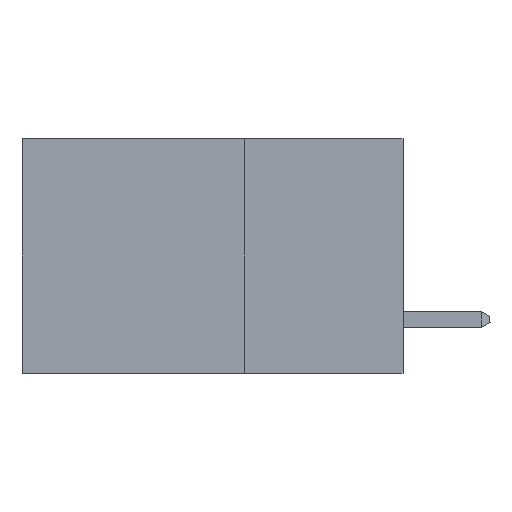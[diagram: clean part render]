
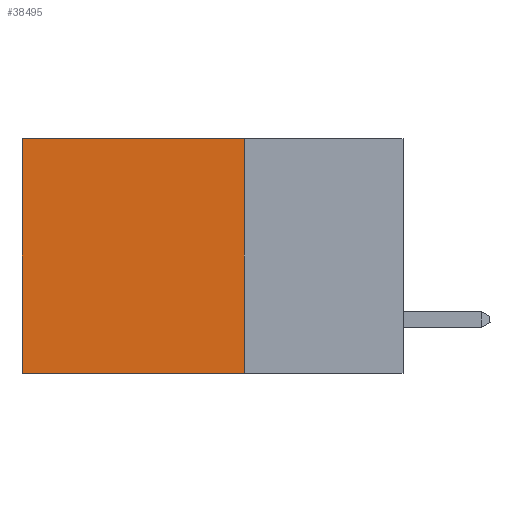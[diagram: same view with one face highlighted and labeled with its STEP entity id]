
A CAD part, left-side view. The second image highlights one B-rep face of the part: STEP entity #38495.
In plain terms, the highlighted planar face has unit normal (-1, 0, 0).
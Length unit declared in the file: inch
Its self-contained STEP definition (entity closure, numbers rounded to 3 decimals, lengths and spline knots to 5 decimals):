
#2037 = PLANE ( 'NONE',  #40340 ) ;
#2055 = CARTESIAN_POINT ( 'NONE',  ( 0.2875, 0.25, 0. ) ) ;
#2786 = VERTEX_POINT ( 'NONE', #8508 ) ;
#3442 = FACE_OUTER_BOUND ( 'NONE', #38806, .T. ) ;
#3471 = CARTESIAN_POINT ( 'NONE',  ( 0.2875, 0.25, 0. ) ) ;
#4425 = VECTOR ( 'NONE', #43375, 39.37008 ) ;
#5122 = EDGE_CURVE ( 'NONE', #25894, #33796, #31458, .T. ) ;
#5838 = CARTESIAN_POINT ( 'NONE',  ( 0.2875, 0.25, 0. ) ) ;
#7731 = CARTESIAN_POINT ( 'NONE',  ( 0.2875, 0.6, 0. ) ) ;
#8087 = ORIENTED_EDGE ( 'NONE', *, *, #5122, .F. ) ;
#8508 = CARTESIAN_POINT ( 'NONE',  ( 0.2875, 0.6, -0.37 ) ) ;
#11336 = VECTOR ( 'NONE', #37614, 39.37008 ) ;
#13285 = DIRECTION ( 'NONE',  ( 1., 0., 0. ) ) ;
#15306 = CARTESIAN_POINT ( 'NONE',  ( 0.2875, 0.25, -0.37 ) ) ;
#16373 = DIRECTION ( 'NONE',  ( 0., 1., 0. ) ) ;
#16949 = DIRECTION ( 'NONE',  ( 0., 0., -1. ) ) ;
#21003 = LINE ( 'NONE', #5838, #4425 ) ;
#25248 = ORIENTED_EDGE ( 'NONE', *, *, #46511, .T. ) ;
#25894 = VERTEX_POINT ( 'NONE', #2055 ) ;
#26436 = VECTOR ( 'NONE', #16373, 39.37008 ) ;
#28484 = CARTESIAN_POINT ( 'NONE',  ( 0.2875, 0.25, 0. ) ) ;
#30358 = VERTEX_POINT ( 'NONE', #7731 ) ;
#31458 = LINE ( 'NONE', #3471, #11336 ) ;
#33796 = VERTEX_POINT ( 'NONE', #15306 ) ;
#33809 = ORIENTED_EDGE ( 'NONE', *, *, #45675, .F. ) ;
#34390 = EDGE_CURVE ( 'NONE', #30358, #2786, #45422, .T. ) ;
#37614 = DIRECTION ( 'NONE',  ( 0., 0., -1. ) ) ;
#38005 = CARTESIAN_POINT ( 'NONE',  ( 0.2875, 0.6, 0. ) ) ;
#38495 = ADVANCED_FACE ( 'NONE', ( #3442 ), #2037, .F. ) ;
#38806 = EDGE_LOOP ( 'NONE', ( #41106, #33809, #8087, #25248 ) ) ;
#39003 = CARTESIAN_POINT ( 'NONE',  ( 0.2875, 0.25, -0.37 ) ) ;
#40340 = AXIS2_PLACEMENT_3D ( 'NONE', #28484, #13285, #16949 ) ;
#41106 = ORIENTED_EDGE ( 'NONE', *, *, #34390, .T. ) ;
#42370 = LINE ( 'NONE', #39003, #26436 ) ;
#43375 = DIRECTION ( 'NONE',  ( 0., 1., 0. ) ) ;
#45422 = LINE ( 'NONE', #38005, #46612 ) ;
#45602 = DIRECTION ( 'NONE',  ( 0., 0., -1. ) ) ;
#45675 = EDGE_CURVE ( 'NONE', #33796, #2786, #42370, .T. ) ;
#46511 = EDGE_CURVE ( 'NONE', #25894, #30358, #21003, .T. ) ;
#46612 = VECTOR ( 'NONE', #45602, 39.37008 ) ;
